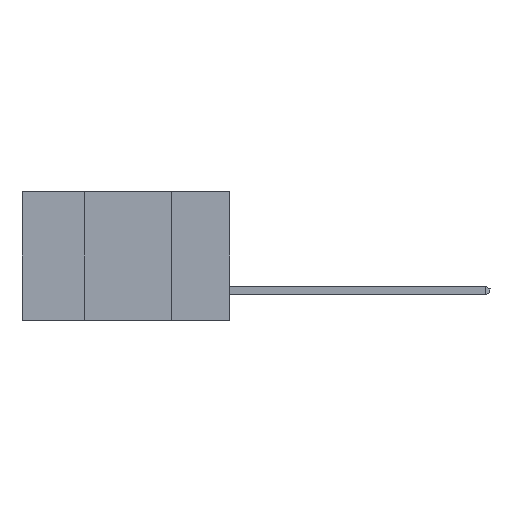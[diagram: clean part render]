
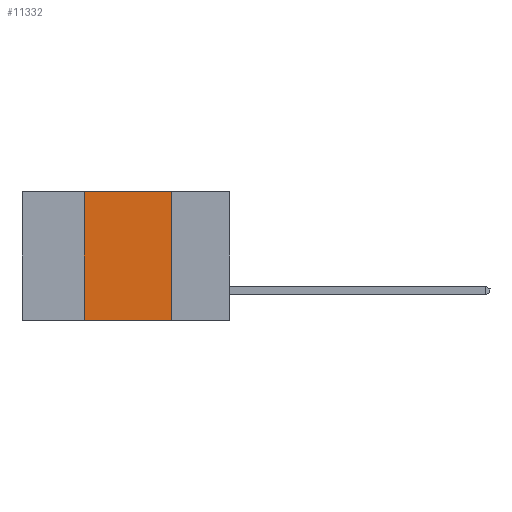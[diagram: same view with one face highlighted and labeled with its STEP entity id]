
A CAD part, left-side view. The second image highlights one B-rep face of the part: STEP entity #11332.
In plain terms, the highlighted planar face has unit normal (-1, 0, 0).
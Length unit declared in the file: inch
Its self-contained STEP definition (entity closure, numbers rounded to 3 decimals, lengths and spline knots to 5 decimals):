
#339 = ORIENTED_EDGE ( 'NONE', *, *, #16403, .T. ) ;
#426 = DIRECTION ( 'NONE',  ( 0., 0., 1. ) ) ;
#438 = DIRECTION ( 'NONE',  ( 0., 0., -1. ) ) ;
#799 = CARTESIAN_POINT ( 'NONE',  ( 0., 0.42, 0. ) ) ;
#925 = AXIS2_PLACEMENT_3D ( 'NONE', #13626, #20126, #438 ) ;
#1247 = CARTESIAN_POINT ( 'NONE',  ( 0., 0.42, -0.37 ) ) ;
#2223 = FACE_OUTER_BOUND ( 'NONE', #8355, .T. ) ;
#3904 = ORIENTED_EDGE ( 'NONE', *, *, #19316, .F. ) ;
#4955 = EDGE_CURVE ( 'NONE', #16835, #17595, #10298, .T. ) ;
#5309 = VECTOR ( 'NONE', #10564, 39.37008 ) ;
#5695 = VERTEX_POINT ( 'NONE', #16175 ) ;
#6165 = ORIENTED_EDGE ( 'NONE', *, *, #4955, .F. ) ;
#6376 = LINE ( 'NONE', #9668, #18562 ) ;
#6841 = LINE ( 'NONE', #19832, #10520 ) ;
#8355 = EDGE_LOOP ( 'NONE', ( #20071, #3904, #6165, #339 ) ) ;
#8368 = CARTESIAN_POINT ( 'NONE',  ( 0., 0.42, -0.37 ) ) ;
#9668 = CARTESIAN_POINT ( 'NONE',  ( 0., 0.17, -0.37 ) ) ;
#10298 = LINE ( 'NONE', #8368, #10808 ) ;
#10341 = LINE ( 'NONE', #20054, #5309 ) ;
#10433 = VERTEX_POINT ( 'NONE', #13759 ) ;
#10520 = VECTOR ( 'NONE', #16633, 39.37008 ) ;
#10564 = DIRECTION ( 'NONE',  ( 0., -1., 0. ) ) ;
#10808 = VECTOR ( 'NONE', #426, 39.37008 ) ;
#11332 = ADVANCED_FACE ( 'NONE', ( #2223 ), #16710, .F. ) ;
#12420 = EDGE_CURVE ( 'NONE', #5695, #10433, #6376, .T. ) ;
#13626 = CARTESIAN_POINT ( 'NONE',  ( 0., 0.6, 0. ) ) ;
#13759 = CARTESIAN_POINT ( 'NONE',  ( 0., 0.17, -0.37 ) ) ;
#16168 = DIRECTION ( 'NONE',  ( 0., 0., -1. ) ) ;
#16175 = CARTESIAN_POINT ( 'NONE',  ( 0., 0.17, 0. ) ) ;
#16403 = EDGE_CURVE ( 'NONE', #16835, #10433, #10341, .T. ) ;
#16633 = DIRECTION ( 'NONE',  ( 0., -1., 0. ) ) ;
#16710 = PLANE ( 'NONE',  #925 ) ;
#16835 = VERTEX_POINT ( 'NONE', #1247 ) ;
#17595 = VERTEX_POINT ( 'NONE', #799 ) ;
#18562 = VECTOR ( 'NONE', #16168, 39.37008 ) ;
#19316 = EDGE_CURVE ( 'NONE', #17595, #5695, #6841, .T. ) ;
#19832 = CARTESIAN_POINT ( 'NONE',  ( 0., 0.6, 0. ) ) ;
#20054 = CARTESIAN_POINT ( 'NONE',  ( 0., 0.6, -0.37 ) ) ;
#20071 = ORIENTED_EDGE ( 'NONE', *, *, #12420, .F. ) ;
#20126 = DIRECTION ( 'NONE',  ( 1., 0., 0. ) ) ;
